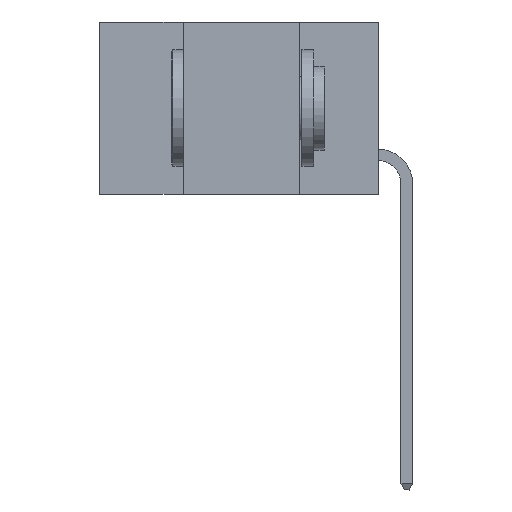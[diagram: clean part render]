
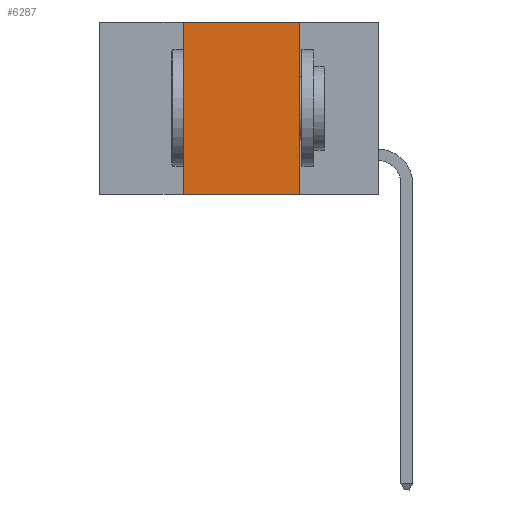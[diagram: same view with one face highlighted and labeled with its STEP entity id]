
A CAD part, left-side view. The second image highlights one B-rep face of the part: STEP entity #6287.
In plain terms, the highlighted planar face has unit normal (-1, 0, 0).
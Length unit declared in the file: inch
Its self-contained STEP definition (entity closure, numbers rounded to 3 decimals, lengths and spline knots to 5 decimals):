
#780 = ORIENTED_EDGE ( 'NONE', *, *, #11660, .F. ) ;
#1180 = VERTEX_POINT ( 'NONE', #14090 ) ;
#2320 = PLANE ( 'NONE',  #12662 ) ;
#2405 = DIRECTION ( 'NONE',  ( 0., 0., -1. ) ) ;
#2593 = ORIENTED_EDGE ( 'NONE', *, *, #12717, .F. ) ;
#3371 = CARTESIAN_POINT ( 'NONE',  ( 0., 0.6, -0.37 ) ) ;
#3885 = VECTOR ( 'NONE', #4963, 39.37008 ) ;
#3952 = ORIENTED_EDGE ( 'NONE', *, *, #6923, .F. ) ;
#4963 = DIRECTION ( 'NONE',  ( 0., -1., 0. ) ) ;
#5327 = FACE_OUTER_BOUND ( 'NONE', #11053, .T. ) ;
#5878 = CARTESIAN_POINT ( 'NONE',  ( 0., 0.42, 0. ) ) ;
#6287 = ADVANCED_FACE ( 'NONE', ( #5327 ), #2320, .F. ) ;
#6923 = EDGE_CURVE ( 'NONE', #1180, #8534, #14423, .T. ) ;
#8152 = CARTESIAN_POINT ( 'NONE',  ( 0., 0.6, 0. ) ) ;
#8534 = VERTEX_POINT ( 'NONE', #17665 ) ;
#8765 = CARTESIAN_POINT ( 'NONE',  ( 0., 0.17, 0. ) ) ;
#9099 = ORIENTED_EDGE ( 'NONE', *, *, #10603, .T. ) ;
#9288 = VERTEX_POINT ( 'NONE', #17904 ) ;
#10021 = VECTOR ( 'NONE', #12218, 39.37008 ) ;
#10300 = CARTESIAN_POINT ( 'NONE',  ( 0., 0.42, -0.37 ) ) ;
#10358 = DIRECTION ( 'NONE',  ( 0., -1., 0. ) ) ;
#10603 = EDGE_CURVE ( 'NONE', #14737, #9288, #20022, .T. ) ;
#11053 = EDGE_LOOP ( 'NONE', ( #2593, #3952, #780, #9099 ) ) ;
#11660 = EDGE_CURVE ( 'NONE', #14737, #1180, #14196, .T. ) ;
#11869 = DIRECTION ( 'NONE',  ( 1., 0., 0. ) ) ;
#12218 = DIRECTION ( 'NONE',  ( 0., 0., 1. ) ) ;
#12662 = AXIS2_PLACEMENT_3D ( 'NONE', #13365, #11869, #2405 ) ;
#12717 = EDGE_CURVE ( 'NONE', #8534, #9288, #18982, .T. ) ;
#13365 = CARTESIAN_POINT ( 'NONE',  ( 0., 0.6, 0. ) ) ;
#13927 = VECTOR ( 'NONE', #10358, 39.37008 ) ;
#14090 = CARTESIAN_POINT ( 'NONE',  ( 0., 0.42, 0. ) ) ;
#14196 = LINE ( 'NONE', #5878, #10021 ) ;
#14423 = LINE ( 'NONE', #8152, #13927 ) ;
#14737 = VERTEX_POINT ( 'NONE', #10300 ) ;
#16547 = DIRECTION ( 'NONE',  ( 0., 0., -1. ) ) ;
#17665 = CARTESIAN_POINT ( 'NONE',  ( 0., 0.17, 0. ) ) ;
#17904 = CARTESIAN_POINT ( 'NONE',  ( 0., 0.17, -0.37 ) ) ;
#18512 = VECTOR ( 'NONE', #16547, 39.37008 ) ;
#18982 = LINE ( 'NONE', #8765, #18512 ) ;
#20022 = LINE ( 'NONE', #3371, #3885 ) ;
